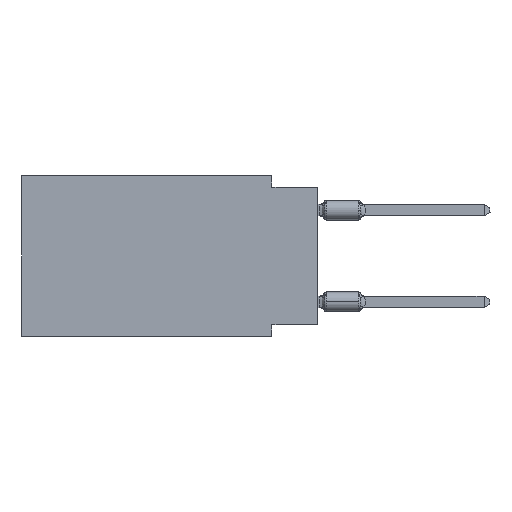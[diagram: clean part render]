
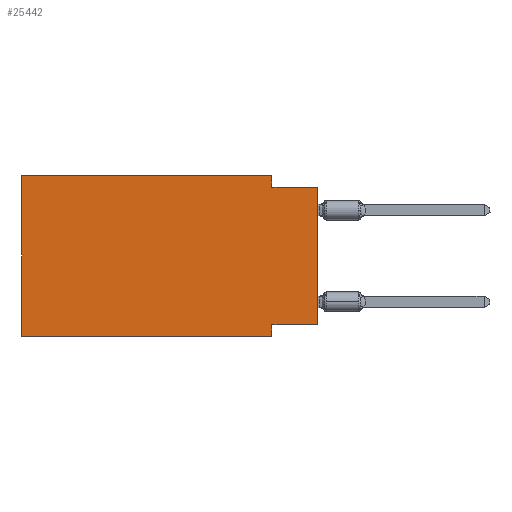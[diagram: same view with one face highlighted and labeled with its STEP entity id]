
A CAD part, left-side view. The second image highlights one B-rep face of the part: STEP entity #25442.
In plain terms, the highlighted planar face has unit normal (-1, 0, 0).
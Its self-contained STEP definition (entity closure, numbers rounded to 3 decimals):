
#283 = CARTESIAN_POINT ( 'NONE',  ( 0., 0., 0. ) ) ;
#779 = CARTESIAN_POINT ( 'NONE',  ( 0., 0., -0.635 ) ) ;
#1218 = CARTESIAN_POINT ( 'NONE',  ( 0., 16.383, -8.89 ) ) ;
#1371 = CARTESIAN_POINT ( 'NONE',  ( 0., 2.54, -8.89 ) ) ;
#1414 = FACE_OUTER_BOUND ( 'NONE', #33785, .T. ) ;
#2468 = EDGE_CURVE ( 'NONE', #10638, #8978, #19733, .T. ) ;
#2996 = LINE ( 'NONE', #283, #28725 ) ;
#3647 = ORIENTED_EDGE ( 'NONE', *, *, #4142, .F. ) ;
#3750 = DIRECTION ( 'NONE',  ( 0., 1., 0. ) ) ;
#4039 = LINE ( 'NONE', #24352, #21665 ) ;
#4142 = EDGE_CURVE ( 'NONE', #33248, #28297, #28619, .T. ) ;
#6325 = LINE ( 'NONE', #18121, #11000 ) ;
#7903 = VECTOR ( 'NONE', #9915, 1000. ) ;
#8600 = ORIENTED_EDGE ( 'NONE', *, *, #19685, .F. ) ;
#8978 = VERTEX_POINT ( 'NONE', #779 ) ;
#9915 = DIRECTION ( 'NONE',  ( 0., -1., 0. ) ) ;
#10323 = VECTOR ( 'NONE', #17933, 1000. ) ;
#10638 = VERTEX_POINT ( 'NONE', #27058 ) ;
#10877 = CARTESIAN_POINT ( 'NONE',  ( 0., 16.383, 0. ) ) ;
#11000 = VECTOR ( 'NONE', #36486, 1000. ) ;
#12719 = DIRECTION ( 'NONE',  ( 0., -1., 0. ) ) ;
#12815 = VERTEX_POINT ( 'NONE', #33350 ) ;
#13663 = VERTEX_POINT ( 'NONE', #14387 ) ;
#13772 = DIRECTION ( 'NONE',  ( 1., 0., 0. ) ) ;
#13910 = DIRECTION ( 'NONE',  ( 0., 0., -1. ) ) ;
#14387 = CARTESIAN_POINT ( 'NONE',  ( 0., 0., -8.255 ) ) ;
#15325 = VERTEX_POINT ( 'NONE', #10877 ) ;
#15733 = CARTESIAN_POINT ( 'NONE',  ( 0., 2.54, -8.89 ) ) ;
#15843 = VECTOR ( 'NONE', #3750, 1000. ) ;
#15915 = LINE ( 'NONE', #1218, #7903 ) ;
#16126 = VERTEX_POINT ( 'NONE', #33236 ) ;
#16657 = EDGE_CURVE ( 'NONE', #13663, #8978, #2996, .T. ) ;
#17684 = DIRECTION ( 'NONE',  ( 0., 0., 1. ) ) ;
#17933 = DIRECTION ( 'NONE',  ( 0., 0., 1. ) ) ;
#18121 = CARTESIAN_POINT ( 'NONE',  ( 0., 2.54, 0. ) ) ;
#18589 = ORIENTED_EDGE ( 'NONE', *, *, #16657, .T. ) ;
#19006 = VECTOR ( 'NONE', #37341, 1000. ) ;
#19012 = CARTESIAN_POINT ( 'NONE',  ( 0., 16.383, 0. ) ) ;
#19685 = EDGE_CURVE ( 'NONE', #13663, #33248, #23853, .T. ) ;
#19733 = LINE ( 'NONE', #28422, #19006 ) ;
#21034 = EDGE_CURVE ( 'NONE', #12815, #28297, #15915, .T. ) ;
#21404 = LINE ( 'NONE', #32616, #10323 ) ;
#21665 = VECTOR ( 'NONE', #12719, 1000. ) ;
#22028 = EDGE_CURVE ( 'NONE', #12815, #15325, #21404, .T. ) ;
#23343 = ORIENTED_EDGE ( 'NONE', *, *, #32524, .F. ) ;
#23853 = LINE ( 'NONE', #35276, #15843 ) ;
#24352 = CARTESIAN_POINT ( 'NONE',  ( 0., 16.383, 0. ) ) ;
#24368 = CARTESIAN_POINT ( 'NONE',  ( 0., 2.54, -8.255 ) ) ;
#25442 = ADVANCED_FACE ( 'NONE', ( #1414 ), #28473, .F. ) ;
#25582 = DIRECTION ( 'NONE',  ( 0., 0., -1. ) ) ;
#26412 = ORIENTED_EDGE ( 'NONE', *, *, #36985, .F. ) ;
#27058 = CARTESIAN_POINT ( 'NONE',  ( 0., 2.54, -0.635 ) ) ;
#27192 = VECTOR ( 'NONE', #13910, 1000. ) ;
#27781 = AXIS2_PLACEMENT_3D ( 'NONE', #19012, #13772, #25582 ) ;
#28146 = ORIENTED_EDGE ( 'NONE', *, *, #21034, .T. ) ;
#28297 = VERTEX_POINT ( 'NONE', #15733 ) ;
#28422 = CARTESIAN_POINT ( 'NONE',  ( 0., 0., -0.635 ) ) ;
#28473 = PLANE ( 'NONE',  #27781 ) ;
#28619 = LINE ( 'NONE', #1371, #27192 ) ;
#28725 = VECTOR ( 'NONE', #17684, 1000. ) ;
#32524 = EDGE_CURVE ( 'NONE', #16126, #10638, #6325, .T. ) ;
#32616 = CARTESIAN_POINT ( 'NONE',  ( 0., 16.383, 0. ) ) ;
#33236 = CARTESIAN_POINT ( 'NONE',  ( 0., 2.54, 0. ) ) ;
#33248 = VERTEX_POINT ( 'NONE', #24368 ) ;
#33350 = CARTESIAN_POINT ( 'NONE',  ( 0., 16.383, -8.89 ) ) ;
#33785 = EDGE_LOOP ( 'NONE', ( #18589, #36303, #23343, #26412, #38098, #28146, #3647, #8600 ) ) ;
#35276 = CARTESIAN_POINT ( 'NONE',  ( 0., 0., -8.255 ) ) ;
#36303 = ORIENTED_EDGE ( 'NONE', *, *, #2468, .F. ) ;
#36486 = DIRECTION ( 'NONE',  ( 0., 0., -1. ) ) ;
#36985 = EDGE_CURVE ( 'NONE', #15325, #16126, #4039, .T. ) ;
#37341 = DIRECTION ( 'NONE',  ( 0., -1., 0. ) ) ;
#38098 = ORIENTED_EDGE ( 'NONE', *, *, #22028, .F. ) ;
